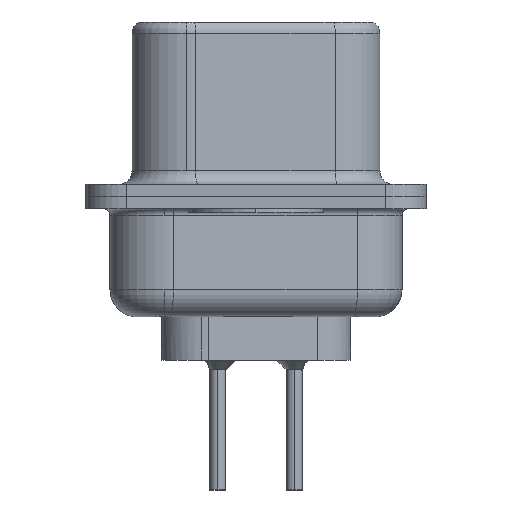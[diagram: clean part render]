
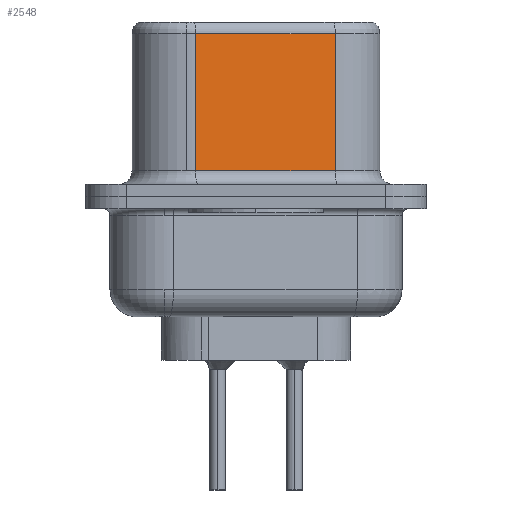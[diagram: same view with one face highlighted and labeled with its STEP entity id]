
A CAD part, left-side view. The second image highlights one B-rep face of the part: STEP entity #2548.
In plain terms, the highlighted planar face has unit normal (-0.985, -0.174, 0).
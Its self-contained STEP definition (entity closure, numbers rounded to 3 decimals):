
#418 = EDGE_CURVE ( 'NONE', #10467, #748, #7606, .T. ) ;
#748 = VERTEX_POINT ( 'NONE', #2553 ) ;
#1375 = DIRECTION ( 'NONE',  ( 0.174, -0.985, 0. ) ) ;
#1815 = ORIENTED_EDGE ( 'NONE', *, *, #7009, .T. ) ;
#2423 = VECTOR ( 'NONE', #16052, 1000. ) ;
#2548 = ADVANCED_FACE ( 'NONE', ( #4361 ), #10405, .F. ) ;
#2553 = CARTESIAN_POINT ( 'NONE',  ( 4.575, -2.927, 0.95 ) ) ;
#2632 = ORIENTED_EDGE ( 'NONE', *, *, #7523, .F. ) ;
#3720 = EDGE_LOOP ( 'NONE', ( #2632, #1815, #4688, #6705 ) ) ;
#4361 = FACE_OUTER_BOUND ( 'NONE', #3720, .T. ) ;
#4467 = DIRECTION ( 'NONE',  ( 0.985, 0.174, 0. ) ) ;
#4688 = ORIENTED_EDGE ( 'NONE', *, *, #9603, .T. ) ;
#5048 = CARTESIAN_POINT ( 'NONE',  ( 3.665, 2.233, 0.95 ) ) ;
#5214 = CARTESIAN_POINT ( 'NONE',  ( 3.665, 2.233, 6.02 ) ) ;
#5225 = VECTOR ( 'NONE', #1375, 1000. ) ;
#5451 = LINE ( 'NONE', #8232, #5877 ) ;
#5877 = VECTOR ( 'NONE', #11393, 1000. ) ;
#6705 = ORIENTED_EDGE ( 'NONE', *, *, #418, .T. ) ;
#7009 = EDGE_CURVE ( 'NONE', #9957, #12211, #16974, .T. ) ;
#7523 = EDGE_CURVE ( 'NONE', #9957, #748, #15949, .T. ) ;
#7606 = LINE ( 'NONE', #8787, #5225 ) ;
#7992 = DIRECTION ( 'NONE',  ( -0.174, 0.985, 0. ) ) ;
#8232 = CARTESIAN_POINT ( 'NONE',  ( 3.665, 2.233, 6.52 ) ) ;
#8787 = CARTESIAN_POINT ( 'NONE',  ( 4.575, -2.927, 0.95 ) ) ;
#8928 = CARTESIAN_POINT ( 'NONE',  ( 4.575, -2.927, 6.52 ) ) ;
#9100 = CARTESIAN_POINT ( 'NONE',  ( 4.575, -2.927, 6.02 ) ) ;
#9486 = CARTESIAN_POINT ( 'NONE',  ( 4.575, -2.927, 6.02 ) ) ;
#9603 = EDGE_CURVE ( 'NONE', #12211, #10467, #5451, .T. ) ;
#9957 = VERTEX_POINT ( 'NONE', #9100 ) ;
#10405 = PLANE ( 'NONE',  #15774 ) ;
#10467 = VERTEX_POINT ( 'NONE', #5048 ) ;
#11393 = DIRECTION ( 'NONE',  ( 0., 0., -1. ) ) ;
#12211 = VERTEX_POINT ( 'NONE', #5214 ) ;
#13466 = DIRECTION ( 'NONE',  ( -0.174, 0.985, 0. ) ) ;
#13760 = VECTOR ( 'NONE', #7992, 1000. ) ;
#14485 = CARTESIAN_POINT ( 'NONE',  ( 4.575, -2.927, 6.52 ) ) ;
#15774 = AXIS2_PLACEMENT_3D ( 'NONE', #8928, #4467, #13466 ) ;
#15949 = LINE ( 'NONE', #14485, #2423 ) ;
#16052 = DIRECTION ( 'NONE',  ( 0., 0., -1. ) ) ;
#16974 = LINE ( 'NONE', #9486, #13760 ) ;
